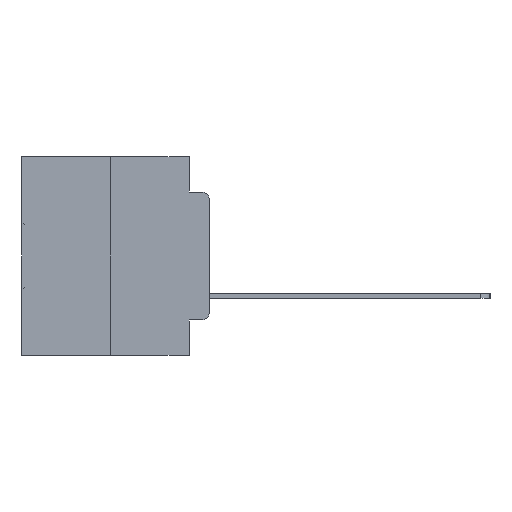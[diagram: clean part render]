
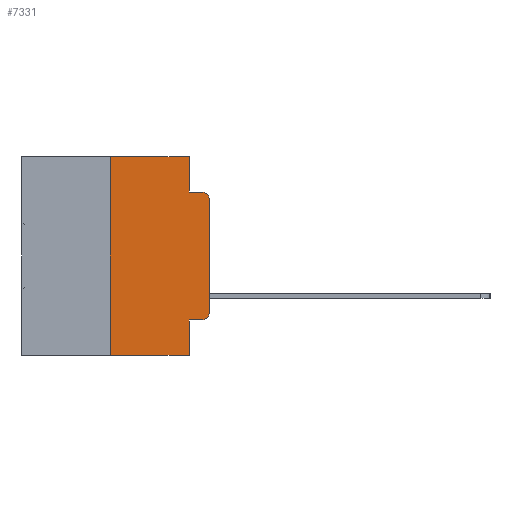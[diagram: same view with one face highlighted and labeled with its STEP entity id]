
A CAD part, left-side view. The second image highlights one B-rep face of the part: STEP entity #7331.
In plain terms, the highlighted planar face has unit normal (-1, 0, 0).
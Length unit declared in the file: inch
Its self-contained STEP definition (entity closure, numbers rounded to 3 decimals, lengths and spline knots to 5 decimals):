
#87 = AXIS2_PLACEMENT_3D ( 'NONE', #12416, #29655, #14964 ) ;
#120 = EDGE_CURVE ( 'NONE', #9270, #4380, #599, .T. ) ;
#539 = DIRECTION ( 'NONE',  ( 0., 0., -1. ) ) ;
#597 = VERTEX_POINT ( 'NONE', #16232 ) ;
#599 = LINE ( 'NONE', #1216, #26675 ) ;
#623 = EDGE_LOOP ( 'NONE', ( #9292, #10902, #11720, #11942, #13405, #14396, #15549, #15648, #16302, #16402 ) ) ;
#1216 = CARTESIAN_POINT ( 'NONE',  ( 0., 0.051, 0. ) ) ;
#1225 = EDGE_CURVE ( 'NONE', #9575, #9384, #28490, .T. ) ;
#1785 = DIRECTION ( 'NONE',  ( 0., 0., -1. ) ) ;
#1988 = DIRECTION ( 'NONE',  ( 0., -1., 0. ) ) ;
#2672 = LINE ( 'NONE', #4493, #28577 ) ;
#2690 = DIRECTION ( 'NONE',  ( -1., 0., 0. ) ) ;
#3213 = LINE ( 'NONE', #11024, #21838 ) ;
#4380 = VERTEX_POINT ( 'NONE', #15236 ) ;
#4493 = CARTESIAN_POINT ( 'NONE',  ( 0., 0.051, -0.4115 ) ) ;
#5183 = CIRCLE ( 'NONE', #6888, 0.02 ) ;
#6271 = CARTESIAN_POINT ( 'NONE',  ( 0., 0.25, 0. ) ) ;
#6888 = AXIS2_PLACEMENT_3D ( 'NONE', #17977, #2690, #20478 ) ;
#7331 = ADVANCED_FACE ( 'NONE', ( #17823 ), #29777, .F. ) ;
#8398 = DIRECTION ( 'NONE',  ( 0., -1., 0. ) ) ;
#8855 = CARTESIAN_POINT ( 'NONE',  ( 0., 0.25, -0.5 ) ) ;
#8863 = EDGE_CURVE ( 'NONE', #9501, #18294, #13151, .T. ) ;
#9270 = VERTEX_POINT ( 'NONE', #20519 ) ;
#9285 = CARTESIAN_POINT ( 'NONE',  ( 0., 0., 0. ) ) ;
#9292 = ORIENTED_EDGE ( 'NONE', *, *, #1225, .T. ) ;
#9384 = VERTEX_POINT ( 'NONE', #30612 ) ;
#9501 = VERTEX_POINT ( 'NONE', #8855 ) ;
#9575 = VERTEX_POINT ( 'NONE', #28919 ) ;
#10856 = CARTESIAN_POINT ( 'NONE',  ( 0., 0.473, -0.5 ) ) ;
#10902 = ORIENTED_EDGE ( 'NONE', *, *, #27200, .T. ) ;
#11024 = CARTESIAN_POINT ( 'NONE',  ( 0., 0.473, 0. ) ) ;
#11720 = ORIENTED_EDGE ( 'NONE', *, *, #19007, .F. ) ;
#11942 = ORIENTED_EDGE ( 'NONE', *, *, #15685, .F. ) ;
#12276 = CARTESIAN_POINT ( 'NONE',  ( 0., 0.051, 0. ) ) ;
#12416 = CARTESIAN_POINT ( 'NONE',  ( 0., 0.02, -0.1085 ) ) ;
#12967 = VECTOR ( 'NONE', #539, 39.37008 ) ;
#13151 = LINE ( 'NONE', #6271, #19046 ) ;
#13405 = ORIENTED_EDGE ( 'NONE', *, *, #13820, .F. ) ;
#13820 = EDGE_CURVE ( 'NONE', #18294, #29847, #3213, .T. ) ;
#14396 = ORIENTED_EDGE ( 'NONE', *, *, #8863, .F. ) ;
#14964 = DIRECTION ( 'NONE',  ( 0., 0., -1. ) ) ;
#15093 = DIRECTION ( 'NONE',  ( 0., -1., 0. ) ) ;
#15103 = DIRECTION ( 'NONE',  ( 1., 0., 0. ) ) ;
#15236 = CARTESIAN_POINT ( 'NONE',  ( 0., 0.051, -0.5 ) ) ;
#15549 = ORIENTED_EDGE ( 'NONE', *, *, #17571, .T. ) ;
#15648 = ORIENTED_EDGE ( 'NONE', *, *, #120, .F. ) ;
#15685 = EDGE_CURVE ( 'NONE', #29847, #597, #19640, .T. ) ;
#15979 = CIRCLE ( 'NONE', #87, 0.02 ) ;
#16183 = CARTESIAN_POINT ( 'NONE',  ( 0., 0.02, -0.4115 ) ) ;
#16232 = CARTESIAN_POINT ( 'NONE',  ( 0., 0.051, -0.0885 ) ) ;
#16302 = ORIENTED_EDGE ( 'NONE', *, *, #27803, .T. ) ;
#16402 = ORIENTED_EDGE ( 'NONE', *, *, #17940, .T. ) ;
#16415 = LINE ( 'NONE', #10856, #27902 ) ;
#16693 = VECTOR ( 'NONE', #15093, 39.37008 ) ;
#17571 = EDGE_CURVE ( 'NONE', #9501, #4380, #16415, .T. ) ;
#17823 = FACE_OUTER_BOUND ( 'NONE', #623, .T. ) ;
#17940 = EDGE_CURVE ( 'NONE', #21026, #9575, #5183, .T. ) ;
#17977 = CARTESIAN_POINT ( 'NONE',  ( 0., 0.02, -0.3915 ) ) ;
#18294 = VERTEX_POINT ( 'NONE', #26763 ) ;
#19007 = EDGE_CURVE ( 'NONE', #597, #20581, #29695, .T. ) ;
#19046 = VECTOR ( 'NONE', #31156, 39.37008 ) ;
#19255 = DIRECTION ( 'NONE',  ( 0., 0., 1. ) ) ;
#19640 = LINE ( 'NONE', #25763, #12967 ) ;
#20478 = DIRECTION ( 'NONE',  ( 0., 0., -1. ) ) ;
#20519 = CARTESIAN_POINT ( 'NONE',  ( 0., 0.051, -0.4115 ) ) ;
#20581 = VERTEX_POINT ( 'NONE', #26212 ) ;
#21026 = VERTEX_POINT ( 'NONE', #16183 ) ;
#21838 = VECTOR ( 'NONE', #30749, 39.37008 ) ;
#22021 = VECTOR ( 'NONE', #19255, 39.37008 ) ;
#22475 = CARTESIAN_POINT ( 'NONE',  ( 0., 0.473, 0. ) ) ;
#24439 = AXIS2_PLACEMENT_3D ( 'NONE', #22475, #15103, #32208 ) ;
#25763 = CARTESIAN_POINT ( 'NONE',  ( 0., 0.051, 0. ) ) ;
#26212 = CARTESIAN_POINT ( 'NONE',  ( 0., 0.02, -0.0885 ) ) ;
#26675 = VECTOR ( 'NONE', #1785, 39.37008 ) ;
#26763 = CARTESIAN_POINT ( 'NONE',  ( 0., 0.25, 0. ) ) ;
#27200 = EDGE_CURVE ( 'NONE', #9384, #20581, #15979, .T. ) ;
#27803 = EDGE_CURVE ( 'NONE', #9270, #21026, #2672, .T. ) ;
#27902 = VECTOR ( 'NONE', #8398, 39.37008 ) ;
#28490 = LINE ( 'NONE', #9285, #22021 ) ;
#28577 = VECTOR ( 'NONE', #1988, 39.37008 ) ;
#28919 = CARTESIAN_POINT ( 'NONE',  ( 0., 0., -0.3915 ) ) ;
#29655 = DIRECTION ( 'NONE',  ( -1., 0., 0. ) ) ;
#29695 = LINE ( 'NONE', #32199, #16693 ) ;
#29777 = PLANE ( 'NONE',  #24439 ) ;
#29847 = VERTEX_POINT ( 'NONE', #12276 ) ;
#30612 = CARTESIAN_POINT ( 'NONE',  ( 0., 0., -0.1085 ) ) ;
#30749 = DIRECTION ( 'NONE',  ( 0., -1., 0. ) ) ;
#31156 = DIRECTION ( 'NONE',  ( 0., 0., 1. ) ) ;
#32199 = CARTESIAN_POINT ( 'NONE',  ( 0., 0.051, -0.0885 ) ) ;
#32208 = DIRECTION ( 'NONE',  ( 0., 0., -1. ) ) ;
